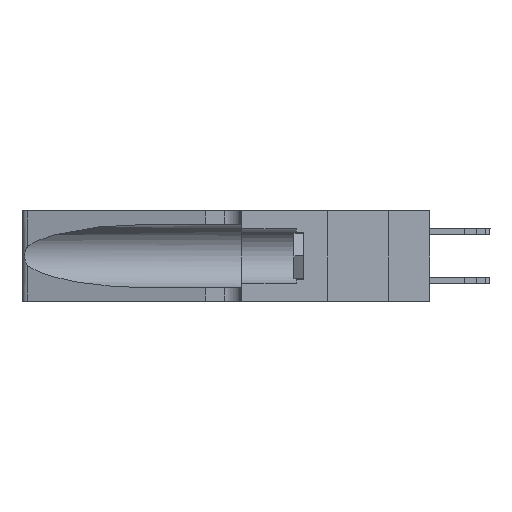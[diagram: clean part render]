
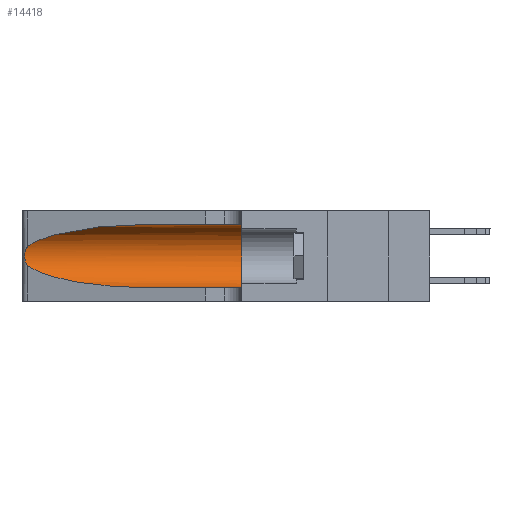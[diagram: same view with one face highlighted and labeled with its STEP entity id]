
A CAD part, left-side view. The second image highlights one B-rep face of the part: STEP entity #14418.
In plain terms, the highlighted cylindrical face has radius 3.308 mm (diameter 6.617 mm), a partial arc.
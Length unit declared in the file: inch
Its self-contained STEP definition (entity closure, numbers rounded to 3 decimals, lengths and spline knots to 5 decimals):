
#68 = CARTESIAN_POINT ( 'NONE',  ( 0.1305, 1.61858, 0.185 ) ) ;
#208 = VERTEX_POINT ( 'NONE', #16321 ) ;
#485 = B_SPLINE_CURVE_WITH_KNOTS ( 'NONE', 3,
 ( #20235, #18818, #18618, #9245, #11005, #15562, #14012, #9514, #9304, #15496, #1966, #7750, #6348, #6232 ),
 .UNSPECIFIED., .F., .F.,
 ( 4, 2, 2, 2, 2, 2, 4 ),
 ( 0., 0.00027, 0.00053, 0.00107, 0.0016, 0.00187, 0.00214 ),
 .UNSPECIFIED. ) ;
#534 = CARTESIAN_POINT ( 'NONE',  ( 0.1305, 0.72297, 0.31525 ) ) ;
#1151 = AXIS2_PLACEMENT_3D ( 'NONE', #16159, #3605, #6687 ) ;
#1164 = DIRECTION ( 'NONE',  ( 0., -1., 0. ) ) ;
#1762 = EDGE_CURVE ( 'NONE', #208, #7856, #4121, .T. ) ;
#1966 = CARTESIAN_POINT ( 'NONE',  ( 0.25789, 1.23486, 0.15765 ) ) ;
#2189 = EDGE_CURVE ( 'NONE', #10563, #2636, #17495, .T. ) ;
#2516 = LINE ( 'NONE', #12552, #16455 ) ;
#2636 = VERTEX_POINT ( 'NONE', #10138 ) ;
#3605 = DIRECTION ( 'NONE',  ( 0., 1., 0. ) ) ;
#3847 = CARTESIAN_POINT ( 'NONE',  ( 0.18966, 0.96281, 0.31525 ) ) ;
#3984 = CARTESIAN_POINT ( 'NONE',  ( 0.25487, 1.22718, 0.22369 ) ) ;
#4121 =( BOUNDED_CURVE ( )  B_SPLINE_CURVE ( 3, ( #6937, #9768, #12952, #16198 ),
 .UNSPECIFIED., .F., .F. ) 
 B_SPLINE_CURVE_WITH_KNOTS ( ( 4, 4 ),
 ( 3.44316, 4.71239 ),
 .UNSPECIFIED. ) 
 CURVE ( )  GEOMETRIC_REPRESENTATION_ITEM ( )  RATIONAL_B_SPLINE_CURVE ( ( 1., 0.87, 0.87, 1. ) ) 
 REPRESENTATION_ITEM ( '' )  );
#4190 = VERTEX_POINT ( 'NONE', #5213 ) ;
#4807 = ORIENTED_EDGE ( 'NONE', *, *, #6805, .T. ) ;
#4830 = CARTESIAN_POINT ( 'NONE',  ( 0.1305, 0.35, 0.31525 ) ) ;
#5213 = CARTESIAN_POINT ( 'NONE',  ( 0.25487, 1.22718, 0.22369 ) ) ;
#6061 = ORIENTED_EDGE ( 'NONE', *, *, #1762, .T. ) ;
#6232 = CARTESIAN_POINT ( 'NONE',  ( 0.25487, 1.22718, 0.14631 ) ) ;
#6348 = CARTESIAN_POINT ( 'NONE',  ( 0.25555, 1.22993, 0.14849 ) ) ;
#6687 = DIRECTION ( 'NONE',  ( 0., 0., 1. ) ) ;
#6805 = EDGE_CURVE ( 'NONE', #7856, #2636, #17323, .T. ) ;
#6937 = CARTESIAN_POINT ( 'NONE',  ( 0.25487, 1.22718, 0.14631 ) ) ;
#7535 =( BOUNDED_CURVE ( )  B_SPLINE_CURVE ( 3, ( #8592, #3847, #13369, #3984 ),
 .UNSPECIFIED., .F., .F. ) 
 B_SPLINE_CURVE_WITH_KNOTS ( ( 4, 4 ),
 ( 1.5708, 2.84003 ),
 .UNSPECIFIED. ) 
 CURVE ( )  GEOMETRIC_REPRESENTATION_ITEM ( )  RATIONAL_B_SPLINE_CURVE ( ( 1., 0.87, 0.87, 1. ) ) 
 REPRESENTATION_ITEM ( '' )  );
#7750 = CARTESIAN_POINT ( 'NONE',  ( 0.25639, 1.23186, 0.15144 ) ) ;
#7856 = VERTEX_POINT ( 'NONE', #13938 ) ;
#8592 = CARTESIAN_POINT ( 'NONE',  ( 0.1305, 0.72297, 0.31525 ) ) ;
#8812 = ORIENTED_EDGE ( 'NONE', *, *, #15230, .T. ) ;
#9122 = ORIENTED_EDGE ( 'NONE', *, *, #17534, .F. ) ;
#9245 = CARTESIAN_POINT ( 'NONE',  ( 0.25787, 1.23484, 0.2124 ) ) ;
#9251 = CYLINDRICAL_SURFACE ( 'NONE', #17557, 0.13025 ) ;
#9304 = CARTESIAN_POINT ( 'NONE',  ( 0.26017, 1.23833, 0.17102 ) ) ;
#9514 = CARTESIAN_POINT ( 'NONE',  ( 0.26075, 1.23896, 0.178 ) ) ;
#9529 = VECTOR ( 'NONE', #1164, 39.37008 ) ;
#9539 = DIRECTION ( 'NONE',  ( 0., -1., 0. ) ) ;
#9768 = CARTESIAN_POINT ( 'NONE',  ( 0.2373, 1.15595, 0.08982 ) ) ;
#10138 = CARTESIAN_POINT ( 'NONE',  ( 0.1305, 0.35, 0.05475 ) ) ;
#10563 = VERTEX_POINT ( 'NONE', #4830 ) ;
#11005 = CARTESIAN_POINT ( 'NONE',  ( 0.25854, 1.2359, 0.20912 ) ) ;
#12479 = ORIENTED_EDGE ( 'NONE', *, *, #2189, .F. ) ;
#12552 = CARTESIAN_POINT ( 'NONE',  ( 0.1305, 1.61858, 0.31525 ) ) ;
#12844 = EDGE_LOOP ( 'NONE', ( #8812, #18384, #6061, #4807, #12479, #9122 ) ) ;
#12952 = CARTESIAN_POINT ( 'NONE',  ( 0.18966, 0.96281, 0.05475 ) ) ;
#13369 = CARTESIAN_POINT ( 'NONE',  ( 0.2373, 1.15595, 0.28018 ) ) ;
#13893 = DIRECTION ( 'NONE',  ( 0., -1., 0. ) ) ;
#13938 = CARTESIAN_POINT ( 'NONE',  ( 0.1305, 0.72297, 0.05475 ) ) ;
#14012 = CARTESIAN_POINT ( 'NONE',  ( 0.26075, 1.23896, 0.19203 ) ) ;
#14418 = ADVANCED_FACE ( 'NONE', ( #18577 ), #9251, .F. ) ;
#15230 = EDGE_CURVE ( 'NONE', #16272, #4190, #7535, .T. ) ;
#15496 = CARTESIAN_POINT ( 'NONE',  ( 0.25856, 1.23593, 0.16098 ) ) ;
#15562 = CARTESIAN_POINT ( 'NONE',  ( 0.26018, 1.23835, 0.19895 ) ) ;
#16126 = EDGE_CURVE ( 'NONE', #4190, #208, #485, .T. ) ;
#16159 = CARTESIAN_POINT ( 'NONE',  ( 0.1305, 0.35, 0.185 ) ) ;
#16198 = CARTESIAN_POINT ( 'NONE',  ( 0.1305, 0.72297, 0.05475 ) ) ;
#16272 = VERTEX_POINT ( 'NONE', #534 ) ;
#16321 = CARTESIAN_POINT ( 'NONE',  ( 0.25487, 1.22718, 0.14631 ) ) ;
#16455 = VECTOR ( 'NONE', #9539, 39.37008 ) ;
#17208 = CARTESIAN_POINT ( 'NONE',  ( 0.1305, 1.61858, 0.05475 ) ) ;
#17323 = LINE ( 'NONE', #17208, #9529 ) ;
#17495 = CIRCLE ( 'NONE', #1151, 0.13025 ) ;
#17534 = EDGE_CURVE ( 'NONE', #16272, #10563, #2516, .T. ) ;
#17557 = AXIS2_PLACEMENT_3D ( 'NONE', #68, #13893, #20171 ) ;
#18384 = ORIENTED_EDGE ( 'NONE', *, *, #16126, .T. ) ;
#18577 = FACE_OUTER_BOUND ( 'NONE', #12844, .T. ) ;
#18618 = CARTESIAN_POINT ( 'NONE',  ( 0.25639, 1.23184, 0.21858 ) ) ;
#18818 = CARTESIAN_POINT ( 'NONE',  ( 0.25555, 1.22994, 0.2215 ) ) ;
#20171 = DIRECTION ( 'NONE',  ( 0., 0., -1. ) ) ;
#20235 = CARTESIAN_POINT ( 'NONE',  ( 0.25487, 1.22718, 0.22369 ) ) ;
